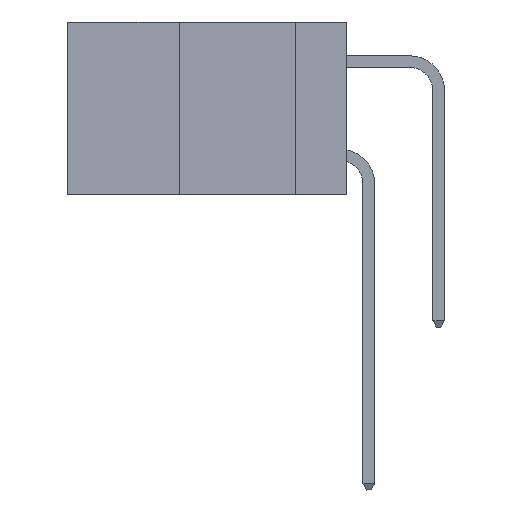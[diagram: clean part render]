
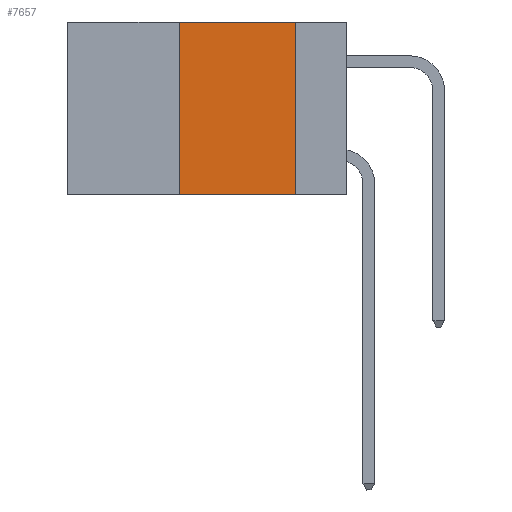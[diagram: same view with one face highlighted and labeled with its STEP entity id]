
A CAD part, left-side view. The second image highlights one B-rep face of the part: STEP entity #7657.
In plain terms, the highlighted planar face has unit normal (-1, 0, 0).
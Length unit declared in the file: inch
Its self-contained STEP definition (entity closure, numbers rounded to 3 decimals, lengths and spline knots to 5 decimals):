
#170 = LINE ( 'NONE', #9144, #12196 ) ;
#282 = CARTESIAN_POINT ( 'NONE',  ( 0., 0.36, -0.37 ) ) ;
#765 = CARTESIAN_POINT ( 'NONE',  ( 0., 0.36, 0. ) ) ;
#1234 = ORIENTED_EDGE ( 'NONE', *, *, #14829, .F. ) ;
#1361 = AXIS2_PLACEMENT_3D ( 'NONE', #10293, #18689, #15314 ) ;
#2150 = VERTEX_POINT ( 'NONE', #16061 ) ;
#3323 = CARTESIAN_POINT ( 'NONE',  ( 0., 0.6, -0.37 ) ) ;
#4988 = VECTOR ( 'NONE', #8324, 39.37008 ) ;
#6025 = LINE ( 'NONE', #3323, #4988 ) ;
#6118 = CARTESIAN_POINT ( 'NONE',  ( 0., 0.36, 0. ) ) ;
#6358 = EDGE_CURVE ( 'NONE', #2150, #15914, #9032, .T. ) ;
#6593 = EDGE_CURVE ( 'NONE', #18722, #9136, #12917, .T. ) ;
#6607 = CARTESIAN_POINT ( 'NONE',  ( 0., 0.11, -0.37 ) ) ;
#6617 = CARTESIAN_POINT ( 'NONE',  ( 0., 0.11, 0. ) ) ;
#7626 = ORIENTED_EDGE ( 'NONE', *, *, #6593, .F. ) ;
#7657 = ADVANCED_FACE ( 'NONE', ( #13667 ), #12245, .F. ) ;
#8324 = DIRECTION ( 'NONE',  ( 0., -1., 0. ) ) ;
#9032 = LINE ( 'NONE', #6617, #13194 ) ;
#9136 = VERTEX_POINT ( 'NONE', #6118 ) ;
#9144 = CARTESIAN_POINT ( 'NONE',  ( 0., 0.6, 0. ) ) ;
#10293 = CARTESIAN_POINT ( 'NONE',  ( 0., 0.6, 0. ) ) ;
#11631 = DIRECTION ( 'NONE',  ( 0., 0., -1. ) ) ;
#12196 = VECTOR ( 'NONE', #16993, 39.37008 ) ;
#12245 = PLANE ( 'NONE',  #1361 ) ;
#12917 = LINE ( 'NONE', #765, #19169 ) ;
#13194 = VECTOR ( 'NONE', #11631, 39.37008 ) ;
#13667 = FACE_OUTER_BOUND ( 'NONE', #14692, .T. ) ;
#14158 = EDGE_CURVE ( 'NONE', #18722, #15914, #6025, .T. ) ;
#14191 = DIRECTION ( 'NONE',  ( 0., 0., 1. ) ) ;
#14692 = EDGE_LOOP ( 'NONE', ( #15660, #1234, #7626, #21292 ) ) ;
#14829 = EDGE_CURVE ( 'NONE', #9136, #2150, #170, .T. ) ;
#15314 = DIRECTION ( 'NONE',  ( 0., 0., -1. ) ) ;
#15660 = ORIENTED_EDGE ( 'NONE', *, *, #6358, .F. ) ;
#15914 = VERTEX_POINT ( 'NONE', #6607 ) ;
#16061 = CARTESIAN_POINT ( 'NONE',  ( 0., 0.11, 0. ) ) ;
#16993 = DIRECTION ( 'NONE',  ( 0., -1., 0. ) ) ;
#18689 = DIRECTION ( 'NONE',  ( 1., 0., 0. ) ) ;
#18722 = VERTEX_POINT ( 'NONE', #282 ) ;
#19169 = VECTOR ( 'NONE', #14191, 39.37008 ) ;
#21292 = ORIENTED_EDGE ( 'NONE', *, *, #14158, .T. ) ;
